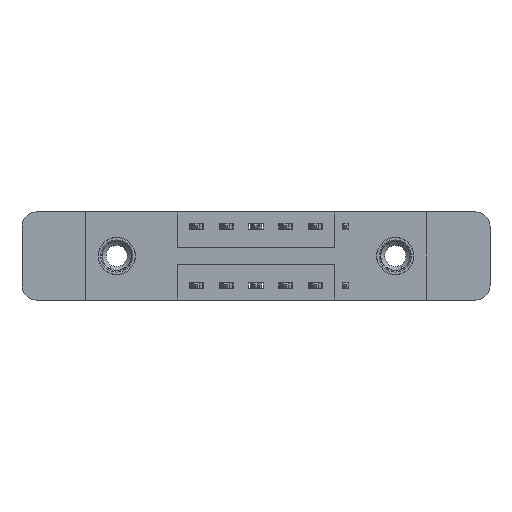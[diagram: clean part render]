
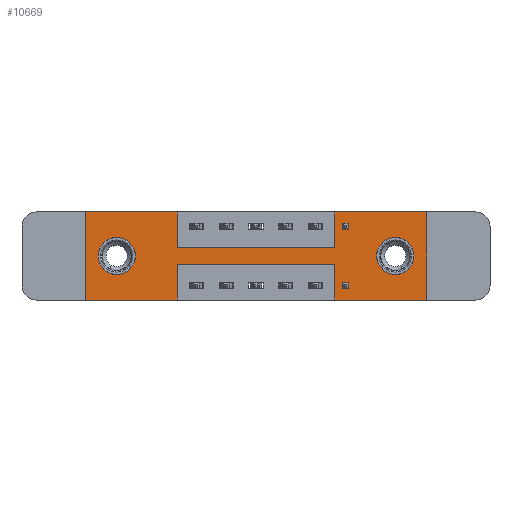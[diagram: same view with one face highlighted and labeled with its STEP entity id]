
A CAD part, front view. The second image highlights one B-rep face of the part: STEP entity #10669.
In plain terms, the highlighted planar face has unit normal (0, -1, 0).
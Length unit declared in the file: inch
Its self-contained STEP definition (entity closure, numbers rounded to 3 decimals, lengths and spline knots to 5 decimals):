
#5 = VERTEX_POINT ( 'NONE', #11197 ) ;
#189 = EDGE_CURVE ( 'NONE', #9840, #4693, #2066, .T. ) ;
#344 = LINE ( 'NONE', #4647, #3675 ) ;
#347 = EDGE_LOOP ( 'NONE', ( #11082, #13032, #3660, #11048, #10700, #2796, #3698, #3585, #3605, #5823, #13895, #2366 ) ) ;
#401 = EDGE_LOOP ( 'NONE', ( #7415, #11552 ) ) ;
#515 = CIRCLE ( 'NONE', #12449, 0.078 ) ;
#591 = CARTESIAN_POINT ( 'NONE',  ( 1.435, 0., 0. ) ) ;
#611 = EDGE_CURVE ( 'NONE', #13900, #12400, #10192, .T. ) ;
#914 = DIRECTION ( 'NONE',  ( -1., 0., 0. ) ) ;
#1196 = VECTOR ( 'NONE', #7533, 39.37008 ) ;
#1217 = EDGE_CURVE ( 'NONE', #6414, #13639, #515, .T. ) ;
#1247 = DIRECTION ( 'NONE',  ( 0., 0., 1. ) ) ;
#1248 = EDGE_CURVE ( 'NONE', #3512, #2707, #344, .T. ) ;
#1328 = EDGE_CURVE ( 'NONE', #13639, #6414, #7284, .T. ) ;
#1346 = VERTEX_POINT ( 'NONE', #13670 ) ;
#1451 = DIRECTION ( 'NONE',  ( 0., 1., 0. ) ) ;
#1511 = EDGE_CURVE ( 'NONE', #13252, #7352, #2289, .T. ) ;
#1633 = CARTESIAN_POINT ( 'NONE',  ( 0., 0., 0. ) ) ;
#1830 = CARTESIAN_POINT ( 'NONE',  ( 0., 0., 0. ) ) ;
#1927 = CARTESIAN_POINT ( 'NONE',  ( 0.3875, 0., -0.22 ) ) ;
#2001 = VERTEX_POINT ( 'NONE', #13564 ) ;
#2066 = LINE ( 'NONE', #3282, #5010 ) ;
#2133 = CARTESIAN_POINT ( 'NONE',  ( 1.0475, 0., -0.15 ) ) ;
#2289 = LINE ( 'NONE', #5214, #1196 ) ;
#2366 = ORIENTED_EDGE ( 'NONE', *, *, #3261, .F. ) ;
#2373 = PLANE ( 'NONE',  #3061 ) ;
#2435 = EDGE_CURVE ( 'NONE', #12400, #9840, #12412, .T. ) ;
#2669 = DIRECTION ( 'NONE',  ( 0., 0., 1. ) ) ;
#2707 = VERTEX_POINT ( 'NONE', #5921 ) ;
#2796 = ORIENTED_EDGE ( 'NONE', *, *, #5679, .F. ) ;
#2899 = DIRECTION ( 'NONE',  ( 1., 0., 0. ) ) ;
#2938 = CARTESIAN_POINT ( 'NONE',  ( 0., 0., 0. ) ) ;
#3061 = AXIS2_PLACEMENT_3D ( 'NONE', #12111, #11111, #12312 ) ;
#3261 = EDGE_CURVE ( 'NONE', #7352, #5219, #6314, .T. ) ;
#3282 = CARTESIAN_POINT ( 'NONE',  ( 1.0475, 0., 0. ) ) ;
#3353 = CIRCLE ( 'NONE', #8302, 0.078 ) ;
#3512 = VERTEX_POINT ( 'NONE', #5952 ) ;
#3517 = VERTEX_POINT ( 'NONE', #3958 ) ;
#3585 = ORIENTED_EDGE ( 'NONE', *, *, #2435, .F. ) ;
#3605 = ORIENTED_EDGE ( 'NONE', *, *, #611, .F. ) ;
#3660 = ORIENTED_EDGE ( 'NONE', *, *, #1248, .F. ) ;
#3675 = VECTOR ( 'NONE', #2669, 39.37008 ) ;
#3698 = ORIENTED_EDGE ( 'NONE', *, *, #189, .F. ) ;
#3705 = VECTOR ( 'NONE', #6382, 39.37008 ) ;
#3714 = FACE_BOUND ( 'NONE', #10383, .T. ) ;
#3882 = VECTOR ( 'NONE', #13002, 39.37008 ) ;
#3885 = VECTOR ( 'NONE', #12348, 39.37008 ) ;
#3939 = CARTESIAN_POINT ( 'NONE',  ( 1.3025, 0., -0.185 ) ) ;
#3958 = CARTESIAN_POINT ( 'NONE',  ( 0.1325, 0., -0.263 ) ) ;
#4153 = VECTOR ( 'NONE', #914, 39.37008 ) ;
#4193 = LINE ( 'NONE', #8484, #3882 ) ;
#4298 = EDGE_CURVE ( 'NONE', #2001, #3512, #11726, .T. ) ;
#4647 = CARTESIAN_POINT ( 'NONE',  ( 1.0475, 0., -0.37 ) ) ;
#4693 = VERTEX_POINT ( 'NONE', #6708 ) ;
#4937 = DIRECTION ( 'NONE',  ( 0., 0., 1. ) ) ;
#5010 = VECTOR ( 'NONE', #5633, 39.37008 ) ;
#5214 = CARTESIAN_POINT ( 'NONE',  ( 0.3875, 0., -0.37 ) ) ;
#5219 = VERTEX_POINT ( 'NONE', #11311 ) ;
#5428 = EDGE_CURVE ( 'NONE', #2707, #13252, #4193, .T. ) ;
#5633 = DIRECTION ( 'NONE',  ( 0., 0., 1. ) ) ;
#5677 = VERTEX_POINT ( 'NONE', #7151 ) ;
#5679 = EDGE_CURVE ( 'NONE', #4693, #5, #12560, .T. ) ;
#5823 = ORIENTED_EDGE ( 'NONE', *, *, #13646, .F. ) ;
#5883 = CARTESIAN_POINT ( 'NONE',  ( 0.3875, 0., -0.37 ) ) ;
#5897 = DIRECTION ( 'NONE',  ( 1., 0., 0. ) ) ;
#5921 = CARTESIAN_POINT ( 'NONE',  ( 1.0475, 0., -0.22 ) ) ;
#5952 = CARTESIAN_POINT ( 'NONE',  ( 1.0475, 0., -0.37 ) ) ;
#6027 = CARTESIAN_POINT ( 'NONE',  ( 0.3875, 0., -0.15 ) ) ;
#6077 = DIRECTION ( 'NONE',  ( 0., 1., 0. ) ) ;
#6145 = CARTESIAN_POINT ( 'NONE',  ( 0.3875, 0., -0.15 ) ) ;
#6314 = LINE ( 'NONE', #10805, #4153 ) ;
#6382 = DIRECTION ( 'NONE',  ( -1., 0., 0. ) ) ;
#6414 = VERTEX_POINT ( 'NONE', #11315 ) ;
#6615 = AXIS2_PLACEMENT_3D ( 'NONE', #3939, #6077, #10293 ) ;
#6695 = FACE_BOUND ( 'NONE', #401, .T. ) ;
#6708 = CARTESIAN_POINT ( 'NONE',  ( 1.0475, 0., 0. ) ) ;
#6916 = CARTESIAN_POINT ( 'NONE',  ( 1.3025, 0., -0.185 ) ) ;
#6981 = DIRECTION ( 'NONE',  ( 0., 0., -1. ) ) ;
#7151 = CARTESIAN_POINT ( 'NONE',  ( 0.1325, 0., -0.107 ) ) ;
#7273 = VECTOR ( 'NONE', #8015, 39.37008 ) ;
#7284 = CIRCLE ( 'NONE', #6615, 0.078 ) ;
#7352 = VERTEX_POINT ( 'NONE', #5883 ) ;
#7415 = ORIENTED_EDGE ( 'NONE', *, *, #1217, .T. ) ;
#7533 = DIRECTION ( 'NONE',  ( 0., 0., -1. ) ) ;
#8015 = DIRECTION ( 'NONE',  ( 0., 0., -1. ) ) ;
#8016 = FACE_OUTER_BOUND ( 'NONE', #347, .T. ) ;
#8302 = AXIS2_PLACEMENT_3D ( 'NONE', #12982, #8600, #12902 ) ;
#8384 = VECTOR ( 'NONE', #2899, 39.37008 ) ;
#8484 = CARTESIAN_POINT ( 'NONE',  ( 0.3875, 0., -0.22 ) ) ;
#8570 = EDGE_CURVE ( 'NONE', #3517, #5677, #3353, .T. ) ;
#8600 = DIRECTION ( 'NONE',  ( 0., 1., 0. ) ) ;
#8640 = VECTOR ( 'NONE', #4937, 39.37008 ) ;
#8885 = DIRECTION ( 'NONE',  ( 0., 1., 0. ) ) ;
#8973 = CARTESIAN_POINT ( 'NONE',  ( 0.3875, 0., 0. ) ) ;
#9367 = LINE ( 'NONE', #2938, #8640 ) ;
#9569 = EDGE_CURVE ( 'NONE', #5677, #3517, #9638, .T. ) ;
#9638 = CIRCLE ( 'NONE', #12335, 0.078 ) ;
#9840 = VERTEX_POINT ( 'NONE', #2133 ) ;
#10192 = LINE ( 'NONE', #12311, #7273 ) ;
#10293 = DIRECTION ( 'NONE',  ( 0., 0., -1. ) ) ;
#10383 = EDGE_LOOP ( 'NONE', ( #13205, #11225 ) ) ;
#10666 = CARTESIAN_POINT ( 'NONE',  ( 0., 0., -0.37 ) ) ;
#10669 = ADVANCED_FACE ( 'NONE', ( #6695, #3714, #8016 ), #2373, .T. ) ;
#10700 = ORIENTED_EDGE ( 'NONE', *, *, #11999, .F. ) ;
#10805 = CARTESIAN_POINT ( 'NONE',  ( 0., 0., -0.37 ) ) ;
#11039 = CARTESIAN_POINT ( 'NONE',  ( 0.1325, 0., -0.185 ) ) ;
#11048 = ORIENTED_EDGE ( 'NONE', *, *, #4298, .F. ) ;
#11082 = ORIENTED_EDGE ( 'NONE', *, *, #1511, .F. ) ;
#11111 = DIRECTION ( 'NONE',  ( 0., -1., 0. ) ) ;
#11197 = CARTESIAN_POINT ( 'NONE',  ( 1.435, 0., 0. ) ) ;
#11225 = ORIENTED_EDGE ( 'NONE', *, *, #8570, .T. ) ;
#11298 = LINE ( 'NONE', #1633, #11577 ) ;
#11311 = CARTESIAN_POINT ( 'NONE',  ( 0., 0., -0.37 ) ) ;
#11315 = CARTESIAN_POINT ( 'NONE',  ( 1.3025, 0., -0.107 ) ) ;
#11520 = DIRECTION ( 'NONE',  ( 0., 0., -1. ) ) ;
#11529 = LINE ( 'NONE', #591, #12656 ) ;
#11552 = ORIENTED_EDGE ( 'NONE', *, *, #1328, .T. ) ;
#11577 = VECTOR ( 'NONE', #5897, 39.37008 ) ;
#11726 = LINE ( 'NONE', #10666, #3705 ) ;
#11999 = EDGE_CURVE ( 'NONE', #5, #2001, #11529, .T. ) ;
#12111 = CARTESIAN_POINT ( 'NONE',  ( 0., 0., -0.37 ) ) ;
#12311 = CARTESIAN_POINT ( 'NONE',  ( 0.3875, 0., 0. ) ) ;
#12312 = DIRECTION ( 'NONE',  ( 0., 0., -1. ) ) ;
#12335 = AXIS2_PLACEMENT_3D ( 'NONE', #11039, #1451, #1247 ) ;
#12348 = DIRECTION ( 'NONE',  ( 1., 0., 0. ) ) ;
#12400 = VERTEX_POINT ( 'NONE', #6145 ) ;
#12412 = LINE ( 'NONE', #6027, #3885 ) ;
#12449 = AXIS2_PLACEMENT_3D ( 'NONE', #6916, #8885, #6981 ) ;
#12560 = LINE ( 'NONE', #1830, #8384 ) ;
#12656 = VECTOR ( 'NONE', #11520, 39.37008 ) ;
#12766 = EDGE_CURVE ( 'NONE', #5219, #1346, #9367, .T. ) ;
#12902 = DIRECTION ( 'NONE',  ( 0., 0., 1. ) ) ;
#12982 = CARTESIAN_POINT ( 'NONE',  ( 0.1325, 0., -0.185 ) ) ;
#13002 = DIRECTION ( 'NONE',  ( -1., 0., 0. ) ) ;
#13032 = ORIENTED_EDGE ( 'NONE', *, *, #5428, .F. ) ;
#13205 = ORIENTED_EDGE ( 'NONE', *, *, #9569, .T. ) ;
#13252 = VERTEX_POINT ( 'NONE', #1927 ) ;
#13564 = CARTESIAN_POINT ( 'NONE',  ( 1.435, 0., -0.37 ) ) ;
#13639 = VERTEX_POINT ( 'NONE', #13698 ) ;
#13646 = EDGE_CURVE ( 'NONE', #1346, #13900, #11298, .T. ) ;
#13670 = CARTESIAN_POINT ( 'NONE',  ( 0., 0., 0. ) ) ;
#13698 = CARTESIAN_POINT ( 'NONE',  ( 1.3025, 0., -0.263 ) ) ;
#13895 = ORIENTED_EDGE ( 'NONE', *, *, #12766, .F. ) ;
#13900 = VERTEX_POINT ( 'NONE', #8973 ) ;
